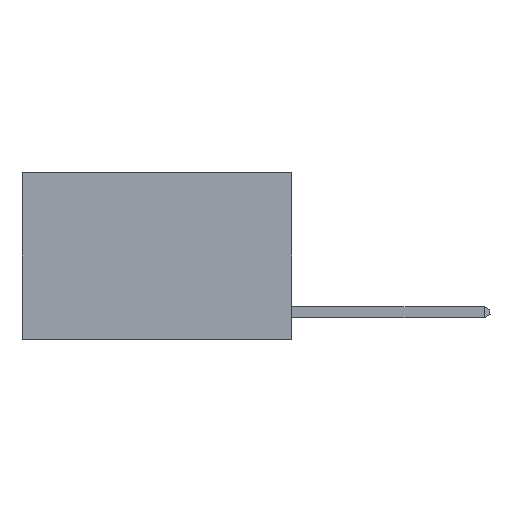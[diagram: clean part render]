
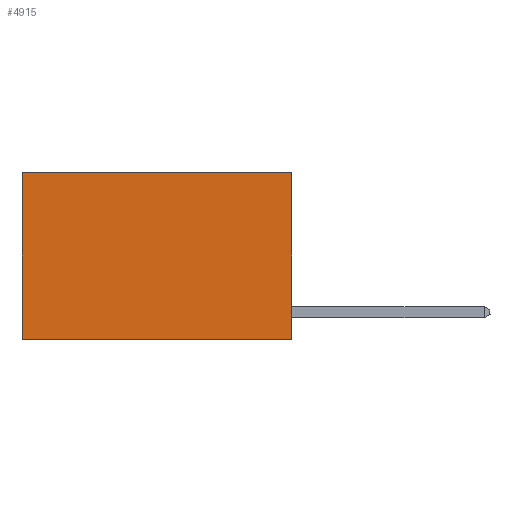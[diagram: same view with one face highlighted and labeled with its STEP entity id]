
A CAD part, left-side view. The second image highlights one B-rep face of the part: STEP entity #4915.
In plain terms, the highlighted planar face has unit normal (-1, 0, 0).
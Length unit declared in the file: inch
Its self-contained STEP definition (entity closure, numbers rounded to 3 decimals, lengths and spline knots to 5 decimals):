
#553 = LINE ( 'NONE', #15016, #21378 ) ;
#590 = PLANE ( 'NONE',  #18082 ) ;
#1279 = CARTESIAN_POINT ( 'NONE',  ( 0.2625, 0., 0. ) ) ;
#1819 = DIRECTION ( 'NONE',  ( 0., 1., 0. ) ) ;
#1891 = ORIENTED_EDGE ( 'NONE', *, *, #3452, .T. ) ;
#2451 = DIRECTION ( 'NONE',  ( 1., 0., 0. ) ) ;
#2687 = ORIENTED_EDGE ( 'NONE', *, *, #14279, .F. ) ;
#2854 = LINE ( 'NONE', #18648, #21745 ) ;
#3150 = LINE ( 'NONE', #1279, #17112 ) ;
#3452 = EDGE_CURVE ( 'NONE', #4163, #15101, #2854, .T. ) ;
#4048 = VERTEX_POINT ( 'NONE', #6705 ) ;
#4095 = ORIENTED_EDGE ( 'NONE', *, *, #13601, .F. ) ;
#4163 = VERTEX_POINT ( 'NONE', #13671 ) ;
#4915 = ADVANCED_FACE ( 'NONE', ( #16446 ), #590, .F. ) ;
#4974 = ORIENTED_EDGE ( 'NONE', *, *, #6322, .T. ) ;
#5884 = CARTESIAN_POINT ( 'NONE',  ( 0.2625, 0., 0. ) ) ;
#6322 = EDGE_CURVE ( 'NONE', #15101, #4048, #553, .T. ) ;
#6705 = CARTESIAN_POINT ( 'NONE',  ( 0.2625, 0.6, -0.37 ) ) ;
#7567 = CARTESIAN_POINT ( 'NONE',  ( 0.2625, 0., -0.37 ) ) ;
#7824 = DIRECTION ( 'NONE',  ( 0., 0., -1. ) ) ;
#8317 = DIRECTION ( 'NONE',  ( 0., 0., -1. ) ) ;
#9228 = DIRECTION ( 'NONE',  ( 0., 0., -1. ) ) ;
#9295 = VECTOR ( 'NONE', #1819, 39.37008 ) ;
#10461 = EDGE_LOOP ( 'NONE', ( #4974, #4095, #2687, #1891 ) ) ;
#10602 = CARTESIAN_POINT ( 'NONE',  ( 0.2625, 0., -0.37 ) ) ;
#12132 = CARTESIAN_POINT ( 'NONE',  ( 0.2625, 0.6, 0. ) ) ;
#12918 = VERTEX_POINT ( 'NONE', #7567 ) ;
#13601 = EDGE_CURVE ( 'NONE', #12918, #4048, #17242, .T. ) ;
#13630 = DIRECTION ( 'NONE',  ( 0., 1., 0. ) ) ;
#13671 = CARTESIAN_POINT ( 'NONE',  ( 0.2625, 0., 0. ) ) ;
#14279 = EDGE_CURVE ( 'NONE', #4163, #12918, #3150, .T. ) ;
#15016 = CARTESIAN_POINT ( 'NONE',  ( 0.2625, 0.6, 0. ) ) ;
#15101 = VERTEX_POINT ( 'NONE', #12132 ) ;
#16446 = FACE_OUTER_BOUND ( 'NONE', #10461, .T. ) ;
#17112 = VECTOR ( 'NONE', #8317, 39.37008 ) ;
#17242 = LINE ( 'NONE', #10602, #9295 ) ;
#18082 = AXIS2_PLACEMENT_3D ( 'NONE', #5884, #2451, #9228 ) ;
#18648 = CARTESIAN_POINT ( 'NONE',  ( 0.2625, 0., 0. ) ) ;
#21378 = VECTOR ( 'NONE', #7824, 39.37008 ) ;
#21745 = VECTOR ( 'NONE', #13630, 39.37008 ) ;
